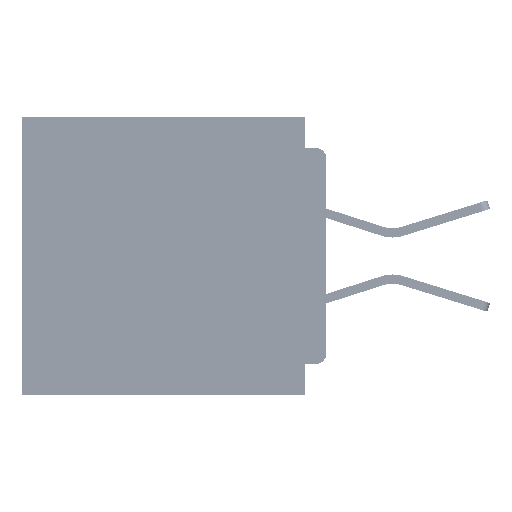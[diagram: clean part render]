
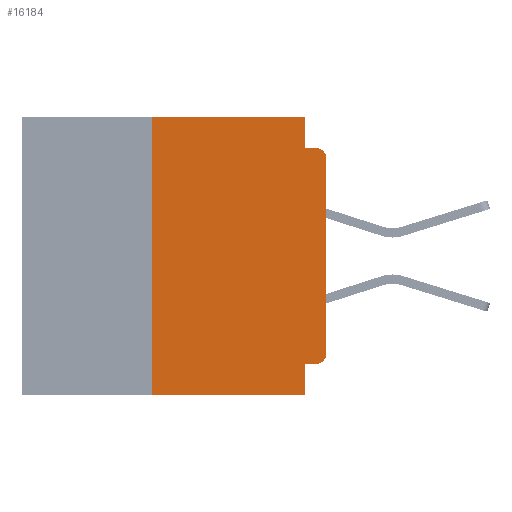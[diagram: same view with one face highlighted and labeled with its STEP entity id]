
A CAD part, left-side view. The second image highlights one B-rep face of the part: STEP entity #16184.
In plain terms, the highlighted planar face has unit normal (-1, 0, 0).
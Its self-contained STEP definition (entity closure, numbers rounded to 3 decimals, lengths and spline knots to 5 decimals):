
#668 = VECTOR ( 'NONE', #14296, 39.37008 ) ;
#2274 = LINE ( 'NONE', #39753, #668 ) ;
#6623 = VERTEX_POINT ( 'NONE', #25361 ) ;
#8205 = CARTESIAN_POINT ( 'NONE',  ( 0., 0.015, -0.355 ) ) ;
#8873 = ORIENTED_EDGE ( 'NONE', *, *, #44259, .T. ) ;
#9179 = DIRECTION ( 'NONE',  ( 0., 0., 1. ) ) ;
#9341 = DIRECTION ( 'NONE',  ( -1., 0., 0. ) ) ;
#10023 = LINE ( 'NONE', #33009, #23565 ) ;
#10474 = EDGE_CURVE ( 'NONE', #12638, #59134, #29400, .T. ) ;
#10917 = CARTESIAN_POINT ( 'NONE',  ( 0., 0.25, 0. ) ) ;
#11009 = CARTESIAN_POINT ( 'NONE',  ( 0., 0.031, -0.045 ) ) ;
#12499 = VECTOR ( 'NONE', #27742, 39.37008 ) ;
#12638 = VERTEX_POINT ( 'NONE', #8205 ) ;
#13008 = VECTOR ( 'NONE', #26384, 39.37008 ) ;
#13483 = LINE ( 'NONE', #56148, #25476 ) ;
#13864 = PLANE ( 'NONE',  #24276 ) ;
#14080 = DIRECTION ( 'NONE',  ( 1., 0., 0. ) ) ;
#14113 = EDGE_CURVE ( 'NONE', #36569, #18798, #13483, .T. ) ;
#14296 = DIRECTION ( 'NONE',  ( 0., 0., -1. ) ) ;
#14605 = CARTESIAN_POINT ( 'NONE',  ( 0., 0.031, 0. ) ) ;
#14631 = VERTEX_POINT ( 'NONE', #27672 ) ;
#16003 = ORIENTED_EDGE ( 'NONE', *, *, #43585, .F. ) ;
#16184 = ADVANCED_FACE ( 'NONE', ( #49224 ), #13864, .F. ) ;
#16223 = LINE ( 'NONE', #41553, #13008 ) ;
#16467 = ORIENTED_EDGE ( 'NONE', *, *, #52958, .F. ) ;
#16677 = CARTESIAN_POINT ( 'NONE',  ( 0., 0., -0.045 ) ) ;
#17446 = CARTESIAN_POINT ( 'NONE',  ( 0., 0.031, -0.4 ) ) ;
#18222 = EDGE_CURVE ( 'NONE', #59134, #29924, #51180, .T. ) ;
#18798 = VERTEX_POINT ( 'NONE', #14605 ) ;
#19946 = EDGE_CURVE ( 'NONE', #29924, #14631, #39919, .T. ) ;
#20640 = ORIENTED_EDGE ( 'NONE', *, *, #61267, .F. ) ;
#21771 = CARTESIAN_POINT ( 'NONE',  ( 0., 0., -0.34 ) ) ;
#22324 = LINE ( 'NONE', #60169, #34324 ) ;
#22563 = ORIENTED_EDGE ( 'NONE', *, *, #18222, .T. ) ;
#23443 = ORIENTED_EDGE ( 'NONE', *, *, #14113, .F. ) ;
#23565 = VECTOR ( 'NONE', #58550, 39.37008 ) ;
#24104 = CARTESIAN_POINT ( 'NONE',  ( 0., 0.437, 0. ) ) ;
#24276 = AXIS2_PLACEMENT_3D ( 'NONE', #24104, #14080, #49765 ) ;
#24299 = CARTESIAN_POINT ( 'NONE',  ( 0., 0.015, -0.34 ) ) ;
#25361 = CARTESIAN_POINT ( 'NONE',  ( 0., 0.031, -0.4 ) ) ;
#25476 = VECTOR ( 'NONE', #25693, 39.37008 ) ;
#25693 = DIRECTION ( 'NONE',  ( 0., -1., 0. ) ) ;
#26384 = DIRECTION ( 'NONE',  ( 0., 1., 0. ) ) ;
#27021 = AXIS2_PLACEMENT_3D ( 'NONE', #24299, #59905, #29466 ) ;
#27672 = CARTESIAN_POINT ( 'NONE',  ( 0., 0.015, -0.045 ) ) ;
#27742 = DIRECTION ( 'NONE',  ( 0., 0., -1. ) ) ;
#29400 = CIRCLE ( 'NONE', #27021, 0.015 ) ;
#29466 = DIRECTION ( 'NONE',  ( 0., 0., -1. ) ) ;
#29924 = VERTEX_POINT ( 'NONE', #35482 ) ;
#32580 = EDGE_CURVE ( 'NONE', #18798, #45284, #2274, .T. ) ;
#33009 = CARTESIAN_POINT ( 'NONE',  ( 0., 0.437, -0.4 ) ) ;
#34324 = VECTOR ( 'NONE', #9179, 39.37008 ) ;
#35292 = EDGE_LOOP ( 'NONE', ( #22563, #35572, #16467, #53760, #23443, #20640, #8873, #16003, #59560, #58012 ) ) ;
#35482 = CARTESIAN_POINT ( 'NONE',  ( 0., 0., -0.06 ) ) ;
#35572 = ORIENTED_EDGE ( 'NONE', *, *, #19946, .T. ) ;
#35881 = CARTESIAN_POINT ( 'NONE',  ( 0., 0.031, -0.355 ) ) ;
#36569 = VERTEX_POINT ( 'NONE', #10917 ) ;
#39272 = VECTOR ( 'NONE', #65795, 39.37008 ) ;
#39753 = CARTESIAN_POINT ( 'NONE',  ( 0., 0.031, 0. ) ) ;
#39919 = CIRCLE ( 'NONE', #53347, 0.015 ) ;
#39921 = CARTESIAN_POINT ( 'NONE',  ( 0., 0.015, -0.06 ) ) ;
#41553 = CARTESIAN_POINT ( 'NONE',  ( 0., 0., -0.355 ) ) ;
#43585 = EDGE_CURVE ( 'NONE', #63870, #6623, #53167, .T. ) ;
#44259 = EDGE_CURVE ( 'NONE', #49804, #6623, #10023, .T. ) ;
#45046 = DIRECTION ( 'NONE',  ( 0., 0., -1. ) ) ;
#45284 = VERTEX_POINT ( 'NONE', #11009 ) ;
#47258 = DIRECTION ( 'NONE',  ( 0., -1., 0. ) ) ;
#49224 = FACE_OUTER_BOUND ( 'NONE', #35292, .T. ) ;
#49765 = DIRECTION ( 'NONE',  ( 0., 0., -1. ) ) ;
#49804 = VERTEX_POINT ( 'NONE', #54514 ) ;
#49860 = EDGE_CURVE ( 'NONE', #12638, #63870, #16223, .T. ) ;
#51180 = LINE ( 'NONE', #60752, #39272 ) ;
#52549 = LINE ( 'NONE', #16677, #65973 ) ;
#52958 = EDGE_CURVE ( 'NONE', #45284, #14631, #52549, .T. ) ;
#53167 = LINE ( 'NONE', #17446, #12499 ) ;
#53347 = AXIS2_PLACEMENT_3D ( 'NONE', #39921, #9341, #45046 ) ;
#53760 = ORIENTED_EDGE ( 'NONE', *, *, #32580, .F. ) ;
#54514 = CARTESIAN_POINT ( 'NONE',  ( 0., 0.25, -0.4 ) ) ;
#56148 = CARTESIAN_POINT ( 'NONE',  ( 0., 0.437, 0. ) ) ;
#58012 = ORIENTED_EDGE ( 'NONE', *, *, #10474, .T. ) ;
#58550 = DIRECTION ( 'NONE',  ( 0., -1., 0. ) ) ;
#59134 = VERTEX_POINT ( 'NONE', #21771 ) ;
#59560 = ORIENTED_EDGE ( 'NONE', *, *, #49860, .F. ) ;
#59905 = DIRECTION ( 'NONE',  ( -1., 0., 0. ) ) ;
#60169 = CARTESIAN_POINT ( 'NONE',  ( 0., 0.25, -0.4 ) ) ;
#60752 = CARTESIAN_POINT ( 'NONE',  ( 0., 0., 0. ) ) ;
#61267 = EDGE_CURVE ( 'NONE', #49804, #36569, #22324, .T. ) ;
#63870 = VERTEX_POINT ( 'NONE', #35881 ) ;
#65795 = DIRECTION ( 'NONE',  ( 0., 0., 1. ) ) ;
#65973 = VECTOR ( 'NONE', #47258, 39.37008 ) ;
